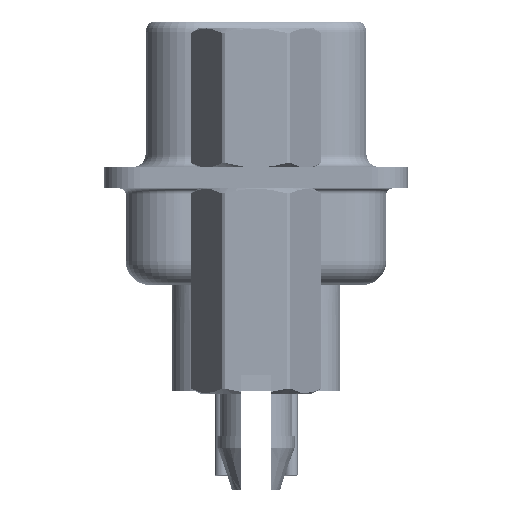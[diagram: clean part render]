
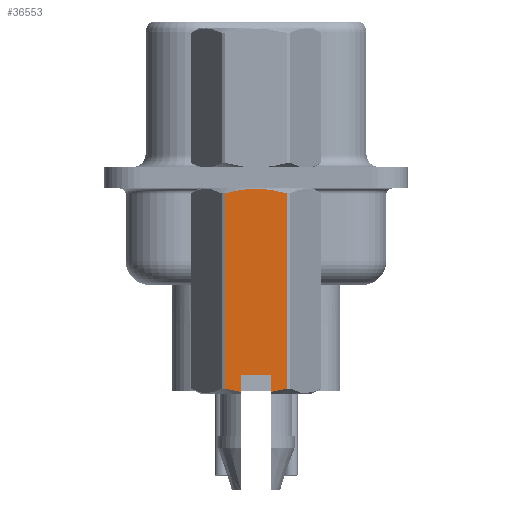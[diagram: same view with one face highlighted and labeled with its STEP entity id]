
A CAD part, left-side view. The second image highlights one B-rep face of the part: STEP entity #36553.
In plain terms, the highlighted planar face has unit normal (-1, 0, 0).
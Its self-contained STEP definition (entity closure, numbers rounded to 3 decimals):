
#2723 = ORIENTED_EDGE ( 'NONE', *, *, #32561, .T. ) ;
#3517 = CARTESIAN_POINT ( 'NONE',  ( -2.381, -1.06, -8.806 ) ) ;
#3983 = CARTESIAN_POINT ( 'NONE',  ( -2.381, 1.066, -0.596 ) ) ;
#6197 = VERTEX_POINT ( 'NONE', #39871 ) ;
#6667 = CARTESIAN_POINT ( 'NONE',  ( -2.381, -1.273, 0.581 ) ) ;
#6813 = CARTESIAN_POINT ( 'NONE',  ( -2.381, -0.625, -8.885 ) ) ;
#7345 = CARTESIAN_POINT ( 'NONE',  ( -2.381, -1.273, -8.748 ) ) ;
#7956 = VERTEX_POINT ( 'NONE', #43674 ) ;
#10997 = CARTESIAN_POINT ( 'NONE',  ( -2.381, 1.273, 0.581 ) ) ;
#11556 = VECTOR ( 'NONE', #46247, 1000. ) ;
#12263 = LINE ( 'NONE', #10997, #45582 ) ;
#12687 = CARTESIAN_POINT ( 'NONE',  ( -2.381, 0.432, -0.485 ) ) ;
#13421 = ORIENTED_EDGE ( 'NONE', *, *, #36730, .T. ) ;
#13505 = B_SPLINE_CURVE_WITH_KNOTS ( 'NONE', 3,
 ( #28156, #47975, #52322, #19478 ),
 .UNSPECIFIED., .F., .F.,
 ( 4, 4 ),
 ( 0.001, 0.002 ),
 .UNSPECIFIED. ) ;
#14206 = VECTOR ( 'NONE', #49861, 1000. ) ;
#14580 = VERTEX_POINT ( 'NONE', #51768 ) ;
#15652 = VERTEX_POINT ( 'NONE', #17391 ) ;
#17391 = CARTESIAN_POINT ( 'NONE',  ( -2.381, -0.625, -8.2 ) ) ;
#19157 = ORIENTED_EDGE ( 'NONE', *, *, #26662, .T. ) ;
#19478 = CARTESIAN_POINT ( 'NONE',  ( -2.381, 0.625, -8.885 ) ) ;
#19556 = CARTESIAN_POINT ( 'NONE',  ( -2.381, -0.842, -8.854 ) ) ;
#20306 = B_SPLINE_CURVE_WITH_KNOTS ( 'NONE', 3,
 ( #45259, #24875, #12687, #41458, #3983, #49589 ),
 .UNSPECIFIED., .F., .F.,
 ( 4, 2, 4 ),
 ( 0.004, 0.004, 0.005 ),
 .UNSPECIFIED. ) ;
#20394 = CARTESIAN_POINT ( 'NONE',  ( -2.381, 0.625, -8.2 ) ) ;
#21024 = CARTESIAN_POINT ( 'NONE',  ( -2.381, 1.273, -8.748 ) ) ;
#21611 = VERTEX_POINT ( 'NONE', #21024 ) ;
#21680 = EDGE_LOOP ( 'NONE', ( #34733, #24194, #2723, #29910, #13421, #44520, #34818, #45105, #19157 ) ) ;
#21809 = LINE ( 'NONE', #46786, #45415 ) ;
#23916 = EDGE_CURVE ( 'NONE', #14580, #41937, #40246, .T. ) ;
#24180 = EDGE_CURVE ( 'NONE', #44901, #45587, #29685, .T. ) ;
#24194 = ORIENTED_EDGE ( 'NONE', *, *, #32084, .F. ) ;
#24875 = CARTESIAN_POINT ( 'NONE',  ( -2.381, 0.215, -0.468 ) ) ;
#26414 = CARTESIAN_POINT ( 'NONE',  ( -2.381, -1.273, -0.652 ) ) ;
#26662 = EDGE_CURVE ( 'NONE', #21611, #45587, #13505, .T. ) ;
#26951 = CARTESIAN_POINT ( 'NONE',  ( -2.381, 0., -0.468 ) ) ;
#28025 = CARTESIAN_POINT ( 'NONE',  ( -2.381, -1.273, -8.748 ) ) ;
#28156 = CARTESIAN_POINT ( 'NONE',  ( -2.381, 1.273, -8.748 ) ) ;
#28440 = CARTESIAN_POINT ( 'NONE',  ( -2.381, -0.625, -8.2 ) ) ;
#29685 = LINE ( 'NONE', #34027, #11556 ) ;
#29910 = ORIENTED_EDGE ( 'NONE', *, *, #23916, .T. ) ;
#30230 = CARTESIAN_POINT ( 'NONE',  ( -2.381, -1.065, -0.596 ) ) ;
#30559 = LINE ( 'NONE', #6667, #41244 ) ;
#31040 = CARTESIAN_POINT ( 'NONE',  ( -2.381, -0.853, -0.549 ) ) ;
#32084 = EDGE_CURVE ( 'NONE', #15652, #44901, #49324, .T. ) ;
#32147 = EDGE_CURVE ( 'NONE', #43916, #7956, #20306, .T. ) ;
#32561 = EDGE_CURVE ( 'NONE', #15652, #14580, #21809, .T. ) ;
#33153 = DIRECTION ( 'NONE',  ( 0., 0., -1. ) ) ;
#33822 = PLANE ( 'NONE',  #42094 ) ;
#34027 = CARTESIAN_POINT ( 'NONE',  ( -2.381, 0.625, -8.2 ) ) ;
#34624 = DIRECTION ( 'NONE',  ( -1., 0., 0. ) ) ;
#34733 = ORIENTED_EDGE ( 'NONE', *, *, #24180, .F. ) ;
#34818 = ORIENTED_EDGE ( 'NONE', *, *, #32147, .T. ) ;
#34833 = CARTESIAN_POINT ( 'NONE',  ( -2.381, -0.428, -0.485 ) ) ;
#34862 = CARTESIAN_POINT ( 'NONE',  ( -2.381, 0., -0.468 ) ) ;
#35247 = EDGE_CURVE ( 'NONE', #7956, #21611, #12263, .T. ) ;
#36553 = ADVANCED_FACE ( 'NONE', ( #38445 ), #33822, .T. ) ;
#36730 = EDGE_CURVE ( 'NONE', #41937, #6197, #30559, .T. ) ;
#38445 = FACE_OUTER_BOUND ( 'NONE', #21680, .T. ) ;
#39785 = DIRECTION ( 'NONE',  ( 0., 0., 1. ) ) ;
#39871 = CARTESIAN_POINT ( 'NONE',  ( -2.381, -1.273, -0.652 ) ) ;
#39905 = EDGE_CURVE ( 'NONE', #6197, #43916, #40143, .T. ) ;
#40143 = B_SPLINE_CURVE_WITH_KNOTS ( 'NONE', 3,
 ( #26414, #30230, #31040, #34833, #51385, #26951 ),
 .UNSPECIFIED., .F., .F.,
 ( 4, 2, 4 ),
 ( 0.003, 0.003, 0.004 ),
 .UNSPECIFIED. ) ;
#40246 = B_SPLINE_CURVE_WITH_KNOTS ( 'NONE', 3,
 ( #6813, #19556, #3517, #7345 ),
 .UNSPECIFIED., .F., .F.,
 ( 4, 4 ),
 ( 0.003, 0.004 ),
 .UNSPECIFIED. ) ;
#41244 = VECTOR ( 'NONE', #39785, 1000. ) ;
#41458 = CARTESIAN_POINT ( 'NONE',  ( -2.381, 0.858, -0.55 ) ) ;
#41716 = DIRECTION ( 'NONE',  ( 0., 0., 1. ) ) ;
#41937 = VERTEX_POINT ( 'NONE', #28025 ) ;
#42094 = AXIS2_PLACEMENT_3D ( 'NONE', #42779, #34624, #41716 ) ;
#42779 = CARTESIAN_POINT ( 'NONE',  ( -2.381, -1.375, 7.399 ) ) ;
#43674 = CARTESIAN_POINT ( 'NONE',  ( -2.381, 1.273, -0.652 ) ) ;
#43916 = VERTEX_POINT ( 'NONE', #34862 ) ;
#44505 = CARTESIAN_POINT ( 'NONE',  ( -2.381, 0.625, -8.885 ) ) ;
#44520 = ORIENTED_EDGE ( 'NONE', *, *, #39905, .T. ) ;
#44901 = VERTEX_POINT ( 'NONE', #20394 ) ;
#45105 = ORIENTED_EDGE ( 'NONE', *, *, #35247, .T. ) ;
#45259 = CARTESIAN_POINT ( 'NONE',  ( -2.381, 0., -0.468 ) ) ;
#45415 = VECTOR ( 'NONE', #50583, 1000. ) ;
#45582 = VECTOR ( 'NONE', #33153, 1000. ) ;
#45587 = VERTEX_POINT ( 'NONE', #44505 ) ;
#46247 = DIRECTION ( 'NONE',  ( 0., 0., -1. ) ) ;
#46786 = CARTESIAN_POINT ( 'NONE',  ( -2.381, -0.625, -8.2 ) ) ;
#47975 = CARTESIAN_POINT ( 'NONE',  ( -2.381, 1.06, -8.806 ) ) ;
#49324 = LINE ( 'NONE', #28440, #14206 ) ;
#49589 = CARTESIAN_POINT ( 'NONE',  ( -2.381, 1.273, -0.652 ) ) ;
#49861 = DIRECTION ( 'NONE',  ( 0., 1., 0. ) ) ;
#50583 = DIRECTION ( 'NONE',  ( 0., 0., -1. ) ) ;
#51385 = CARTESIAN_POINT ( 'NONE',  ( -2.381, -0.215, -0.468 ) ) ;
#51768 = CARTESIAN_POINT ( 'NONE',  ( -2.381, -0.625, -8.885 ) ) ;
#52322 = CARTESIAN_POINT ( 'NONE',  ( -2.381, 0.845, -8.853 ) ) ;
